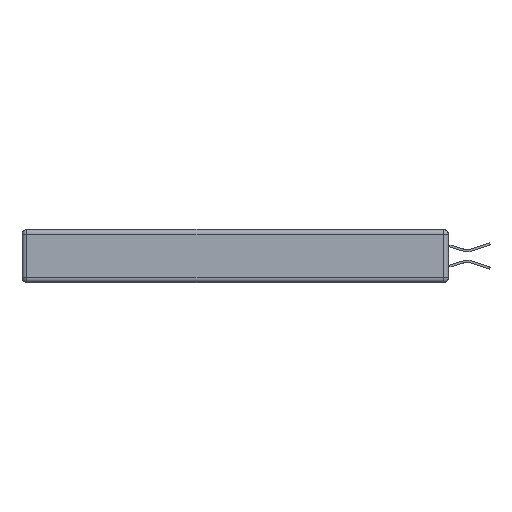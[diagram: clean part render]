
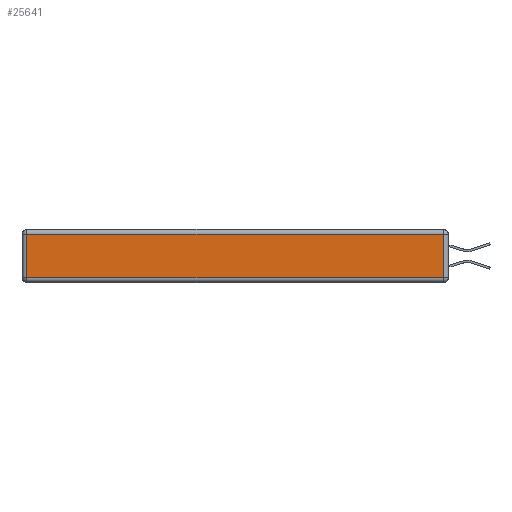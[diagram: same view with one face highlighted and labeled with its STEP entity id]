
A CAD part, left-side view. The second image highlights one B-rep face of the part: STEP entity #25641.
In plain terms, the highlighted planar face has unit normal (-1, 0, 0).
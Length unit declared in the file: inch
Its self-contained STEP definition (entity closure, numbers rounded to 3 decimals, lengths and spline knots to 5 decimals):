
#550 = AXIS2_PLACEMENT_3D ( 'NONE', #24901, #4595, #14641 ) ;
#1989 = LINE ( 'NONE', #2795, #7074 ) ;
#2795 = CARTESIAN_POINT ( 'NONE',  ( 0., 2.75, -0.03 ) ) ;
#3664 = DIRECTION ( 'NONE',  ( 0., 1., 0. ) ) ;
#4595 = DIRECTION ( 'NONE',  ( -1., 0., 0. ) ) ;
#6119 = DIRECTION ( 'NONE',  ( 0., 0., -1. ) ) ;
#6557 = ORIENTED_EDGE ( 'NONE', *, *, #7077, .T. ) ;
#7074 = VECTOR ( 'NONE', #3664, 39.37008 ) ;
#7077 = EDGE_CURVE ( 'NONE', #17668, #26267, #1989, .T. ) ;
#7871 = EDGE_LOOP ( 'NONE', ( #16924, #27358, #6557, #29746 ) ) ;
#9143 = CARTESIAN_POINT ( 'NONE',  ( 0., 2.72, -0.03 ) ) ;
#9696 = CARTESIAN_POINT ( 'NONE',  ( 0., 0.03, -0.03 ) ) ;
#11200 = VECTOR ( 'NONE', #6119, 39.37008 ) ;
#11676 = CARTESIAN_POINT ( 'NONE',  ( 0., 0.03, -0.313 ) ) ;
#12572 = LINE ( 'NONE', #29170, #31061 ) ;
#13740 = CARTESIAN_POINT ( 'NONE',  ( 0., 0.03, -0.343 ) ) ;
#14060 = DIRECTION ( 'NONE',  ( 0., -1., 0. ) ) ;
#14641 = DIRECTION ( 'NONE',  ( 0., 0., 1. ) ) ;
#14961 = PLANE ( 'NONE',  #550 ) ;
#16147 = EDGE_CURVE ( 'NONE', #19568, #17668, #23566, .T. ) ;
#16306 = EDGE_CURVE ( 'NONE', #22192, #19568, #12572, .T. ) ;
#16924 = ORIENTED_EDGE ( 'NONE', *, *, #16306, .T. ) ;
#17668 = VERTEX_POINT ( 'NONE', #9696 ) ;
#18236 = LINE ( 'NONE', #21088, #11200 ) ;
#18277 = EDGE_CURVE ( 'NONE', #26267, #22192, #18236, .T. ) ;
#19568 = VERTEX_POINT ( 'NONE', #11676 ) ;
#21031 = CARTESIAN_POINT ( 'NONE',  ( 0., 2.72, -0.313 ) ) ;
#21088 = CARTESIAN_POINT ( 'NONE',  ( 0., 2.72, -0.343 ) ) ;
#22192 = VERTEX_POINT ( 'NONE', #21031 ) ;
#23566 = LINE ( 'NONE', #13740, #24382 ) ;
#24382 = VECTOR ( 'NONE', #28950, 39.37008 ) ;
#24901 = CARTESIAN_POINT ( 'NONE',  ( 0., 0., -0.343 ) ) ;
#25641 = ADVANCED_FACE ( 'NONE', ( #28251 ), #14961, .T. ) ;
#26267 = VERTEX_POINT ( 'NONE', #9143 ) ;
#27358 = ORIENTED_EDGE ( 'NONE', *, *, #16147, .T. ) ;
#28251 = FACE_OUTER_BOUND ( 'NONE', #7871, .T. ) ;
#28950 = DIRECTION ( 'NONE',  ( 0., 0., 1. ) ) ;
#29170 = CARTESIAN_POINT ( 'NONE',  ( 0., 0., -0.313 ) ) ;
#29746 = ORIENTED_EDGE ( 'NONE', *, *, #18277, .T. ) ;
#31061 = VECTOR ( 'NONE', #14060, 39.37008 ) ;
